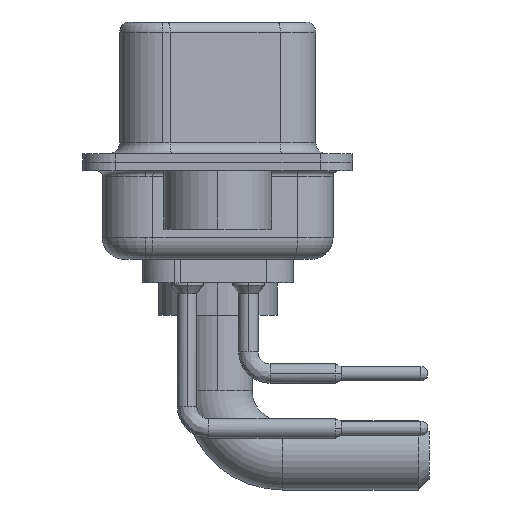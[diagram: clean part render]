
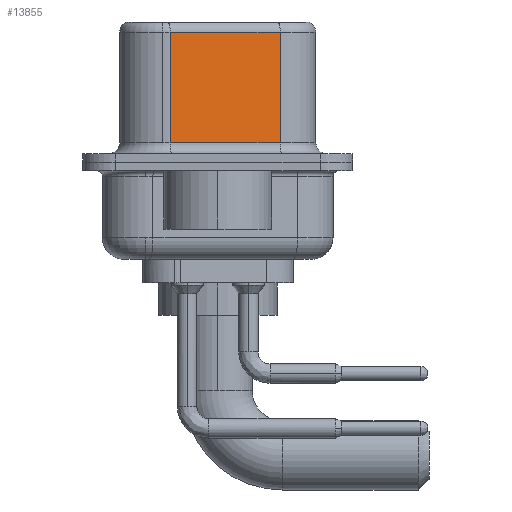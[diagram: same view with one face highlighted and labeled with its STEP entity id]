
A CAD part, left-side view. The second image highlights one B-rep face of the part: STEP entity #13855.
In plain terms, the highlighted planar face has unit normal (-0.985, -0.174, 0).
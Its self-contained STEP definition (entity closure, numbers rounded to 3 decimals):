
#71 = ORIENTED_EDGE ( 'NONE', *, *, #14630, .T. ) ;
#227 = VECTOR ( 'NONE', #12187, 1000. ) ;
#573 = CARTESIAN_POINT ( 'NONE',  ( 3.68, 2.203, 6.52 ) ) ;
#591 = EDGE_CURVE ( 'NONE', #15679, #12025, #6582, .T. ) ;
#900 = DIRECTION ( 'NONE',  ( 0.985, 0.174, 0. ) ) ;
#1228 = LINE ( 'NONE', #11065, #9584 ) ;
#2391 = CARTESIAN_POINT ( 'NONE',  ( 4.58, -2.897, 6.52 ) ) ;
#2724 = VERTEX_POINT ( 'NONE', #9141 ) ;
#4631 = DIRECTION ( 'NONE',  ( 0., 0., -1. ) ) ;
#5409 = DIRECTION ( 'NONE',  ( -0.174, 0.985, 0. ) ) ;
#5561 = EDGE_LOOP ( 'NONE', ( #14120, #11631, #71, #7079 ) ) ;
#6143 = LINE ( 'NONE', #15999, #227 ) ;
#6582 = LINE ( 'NONE', #2391, #10239 ) ;
#7079 = ORIENTED_EDGE ( 'NONE', *, *, #18989, .T. ) ;
#7685 = EDGE_CURVE ( 'NONE', #15679, #17363, #1228, .T. ) ;
#7961 = CARTESIAN_POINT ( 'NONE',  ( 3.68, 2.203, 6.02 ) ) ;
#9141 = CARTESIAN_POINT ( 'NONE',  ( 3.68, 2.203, 0.9 ) ) ;
#9386 = CARTESIAN_POINT ( 'NONE',  ( 4.58, -2.897, 6.02 ) ) ;
#9584 = VECTOR ( 'NONE', #5409, 1000. ) ;
#10131 = VECTOR ( 'NONE', #4631, 1000. ) ;
#10239 = VECTOR ( 'NONE', #22328, 1000. ) ;
#11065 = CARTESIAN_POINT ( 'NONE',  ( 4.58, -2.897, 6.02 ) ) ;
#11631 = ORIENTED_EDGE ( 'NONE', *, *, #7685, .T. ) ;
#12025 = VERTEX_POINT ( 'NONE', #15746 ) ;
#12187 = DIRECTION ( 'NONE',  ( 0.174, -0.985, 0. ) ) ;
#12207 = AXIS2_PLACEMENT_3D ( 'NONE', #15063, #900, #23450 ) ;
#13855 = ADVANCED_FACE ( 'NONE', ( #19126 ), #25406, .F. ) ;
#14120 = ORIENTED_EDGE ( 'NONE', *, *, #591, .F. ) ;
#14630 = EDGE_CURVE ( 'NONE', #17363, #2724, #18558, .T. ) ;
#15063 = CARTESIAN_POINT ( 'NONE',  ( 4.58, -2.897, 6.52 ) ) ;
#15679 = VERTEX_POINT ( 'NONE', #9386 ) ;
#15746 = CARTESIAN_POINT ( 'NONE',  ( 4.58, -2.897, 0.9 ) ) ;
#15999 = CARTESIAN_POINT ( 'NONE',  ( 4.58, -2.897, 0.9 ) ) ;
#17363 = VERTEX_POINT ( 'NONE', #7961 ) ;
#18558 = LINE ( 'NONE', #573, #10131 ) ;
#18989 = EDGE_CURVE ( 'NONE', #2724, #12025, #6143, .T. ) ;
#19126 = FACE_OUTER_BOUND ( 'NONE', #5561, .T. ) ;
#22328 = DIRECTION ( 'NONE',  ( 0., 0., -1. ) ) ;
#23450 = DIRECTION ( 'NONE',  ( -0.174, 0.985, 0. ) ) ;
#25406 = PLANE ( 'NONE',  #12207 ) ;
